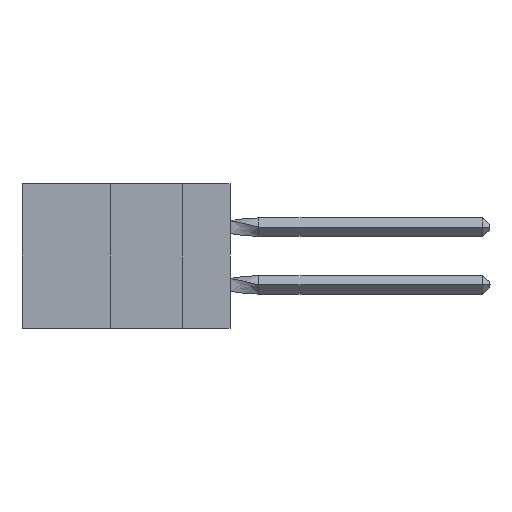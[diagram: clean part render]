
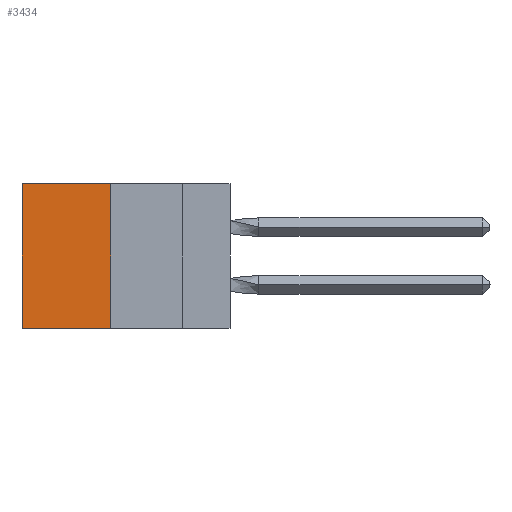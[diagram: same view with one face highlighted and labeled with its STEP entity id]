
A CAD part, left-side view. The second image highlights one B-rep face of the part: STEP entity #3434.
In plain terms, the highlighted planar face has unit normal (-1, 0, 0).
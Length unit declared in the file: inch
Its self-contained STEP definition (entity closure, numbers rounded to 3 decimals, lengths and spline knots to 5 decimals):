
#203 = ORIENTED_EDGE ( 'NONE', *, *, #8894, .F. ) ;
#561 = VERTEX_POINT ( 'NONE', #28491 ) ;
#3434 = ADVANCED_FACE ( 'NONE', ( #4502 ), #4169, .F. ) ;
#3530 = CARTESIAN_POINT ( 'NONE',  ( 0.305, 0.413, -0.5 ) ) ;
#3623 = CARTESIAN_POINT ( 'NONE',  ( 0.305, 0.72, -0.5 ) ) ;
#4169 = PLANE ( 'NONE',  #6465 ) ;
#4462 = VECTOR ( 'NONE', #16232, 39.37008 ) ;
#4502 = FACE_OUTER_BOUND ( 'NONE', #12655, .T. ) ;
#4727 = VECTOR ( 'NONE', #18441, 39.37008 ) ;
#5546 = VERTEX_POINT ( 'NONE', #22034 ) ;
#5837 = CARTESIAN_POINT ( 'NONE',  ( 0.305, 0.413, -0.5 ) ) ;
#6401 = EDGE_CURVE ( 'NONE', #31302, #561, #12958, .T. ) ;
#6465 = AXIS2_PLACEMENT_3D ( 'NONE', #39147, #26410, #13711 ) ;
#8894 = EDGE_CURVE ( 'NONE', #32967, #5546, #9830, .T. ) ;
#9830 = LINE ( 'NONE', #39556, #30569 ) ;
#12655 = EDGE_LOOP ( 'NONE', ( #16970, #203, #15558, #21555 ) ) ;
#12958 = LINE ( 'NONE', #18009, #14992 ) ;
#13711 = DIRECTION ( 'NONE',  ( 0., 0., -1. ) ) ;
#14992 = VECTOR ( 'NONE', #27486, 39.37008 ) ;
#15558 = ORIENTED_EDGE ( 'NONE', *, *, #35455, .F. ) ;
#16232 = DIRECTION ( 'NONE',  ( 0., 0., -1. ) ) ;
#16970 = ORIENTED_EDGE ( 'NONE', *, *, #33670, .T. ) ;
#18009 = CARTESIAN_POINT ( 'NONE',  ( 0.305, 0.413, 0. ) ) ;
#18441 = DIRECTION ( 'NONE',  ( 0., 0., -1. ) ) ;
#18608 = LINE ( 'NONE', #5837, #4727 ) ;
#21555 = ORIENTED_EDGE ( 'NONE', *, *, #6401, .T. ) ;
#22034 = CARTESIAN_POINT ( 'NONE',  ( 0.305, 0.72, -0.5 ) ) ;
#24030 = DIRECTION ( 'NONE',  ( 0., 1., 0. ) ) ;
#26410 = DIRECTION ( 'NONE',  ( 1., 0., 0. ) ) ;
#27486 = DIRECTION ( 'NONE',  ( 0., 1., 0. ) ) ;
#28491 = CARTESIAN_POINT ( 'NONE',  ( 0.305, 0.72, 0. ) ) ;
#30569 = VECTOR ( 'NONE', #24030, 39.37008 ) ;
#31302 = VERTEX_POINT ( 'NONE', #31371 ) ;
#31371 = CARTESIAN_POINT ( 'NONE',  ( 0.305, 0.413, 0. ) ) ;
#32629 = LINE ( 'NONE', #3623, #4462 ) ;
#32967 = VERTEX_POINT ( 'NONE', #3530 ) ;
#33670 = EDGE_CURVE ( 'NONE', #561, #5546, #32629, .T. ) ;
#35455 = EDGE_CURVE ( 'NONE', #31302, #32967, #18608, .T. ) ;
#39147 = CARTESIAN_POINT ( 'NONE',  ( 0.305, 0.413, -0.5 ) ) ;
#39556 = CARTESIAN_POINT ( 'NONE',  ( 0.305, 0.413, -0.5 ) ) ;
